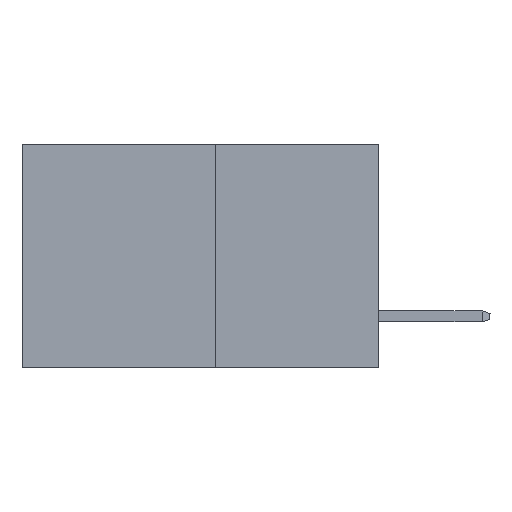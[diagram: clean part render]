
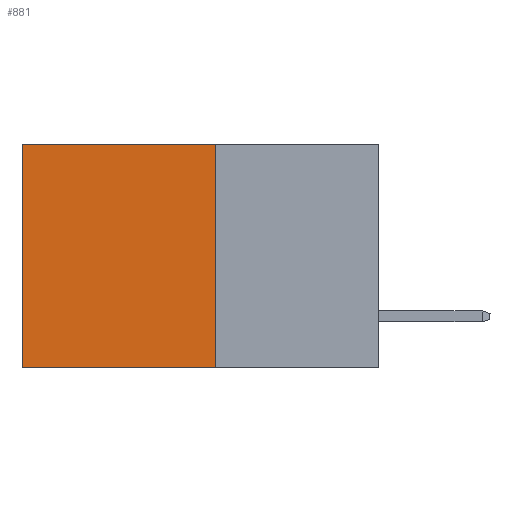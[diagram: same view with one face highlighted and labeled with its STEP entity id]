
A CAD part, left-side view. The second image highlights one B-rep face of the part: STEP entity #881.
In plain terms, the highlighted planar face has unit normal (-1, 0, 0).
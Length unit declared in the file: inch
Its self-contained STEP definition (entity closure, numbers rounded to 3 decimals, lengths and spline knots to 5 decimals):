
#537 = DIRECTION ( 'NONE',  ( 1., 0., 0. ) ) ;
#881 = ADVANCED_FACE ( 'NONE', ( #5533 ), #4506, .F. ) ;
#900 = VECTOR ( 'NONE', #11477, 39.37008 ) ;
#2496 = CARTESIAN_POINT ( 'NONE',  ( 0.277, 0.27, 0. ) ) ;
#2973 = DIRECTION ( 'NONE',  ( 0., 0., -1. ) ) ;
#3085 = DIRECTION ( 'NONE',  ( 0., 0., -1. ) ) ;
#3534 = CARTESIAN_POINT ( 'NONE',  ( 0.277, 0.27, -0.37 ) ) ;
#3695 = ORIENTED_EDGE ( 'NONE', *, *, #5024, .F. ) ;
#3900 = DIRECTION ( 'NONE',  ( 0., 1., 0. ) ) ;
#4506 = PLANE ( 'NONE',  #8404 ) ;
#4558 = CARTESIAN_POINT ( 'NONE',  ( 0.277, 0.27, -0.37 ) ) ;
#5024 = EDGE_CURVE ( 'NONE', #14234, #10140, #5389, .T. ) ;
#5389 = LINE ( 'NONE', #3534, #8649 ) ;
#5533 = FACE_OUTER_BOUND ( 'NONE', #7253, .T. ) ;
#6162 = CARTESIAN_POINT ( 'NONE',  ( 0.277, 0.59, 0. ) ) ;
#6541 = EDGE_CURVE ( 'NONE', #10140, #6581, #16179, .T. ) ;
#6581 = VERTEX_POINT ( 'NONE', #10130 ) ;
#7253 = EDGE_LOOP ( 'NONE', ( #15551, #8063, #3695, #11910 ) ) ;
#8063 = ORIENTED_EDGE ( 'NONE', *, *, #6541, .F. ) ;
#8404 = AXIS2_PLACEMENT_3D ( 'NONE', #4558, #537, #2973 ) ;
#8595 = CARTESIAN_POINT ( 'NONE',  ( 0.277, 0.59, -0.37 ) ) ;
#8649 = VECTOR ( 'NONE', #3085, 39.37008 ) ;
#9406 = EDGE_CURVE ( 'NONE', #14234, #10474, #9484, .T. ) ;
#9484 = LINE ( 'NONE', #2496, #16100 ) ;
#9980 = DIRECTION ( 'NONE',  ( 0., 0., -1. ) ) ;
#10130 = CARTESIAN_POINT ( 'NONE',  ( 0.277, 0.59, -0.37 ) ) ;
#10140 = VERTEX_POINT ( 'NONE', #13617 ) ;
#10474 = VERTEX_POINT ( 'NONE', #6162 ) ;
#11477 = DIRECTION ( 'NONE',  ( 0., 1., 0. ) ) ;
#11517 = EDGE_CURVE ( 'NONE', #10474, #6581, #13441, .T. ) ;
#11769 = CARTESIAN_POINT ( 'NONE',  ( 0.277, 0.27, -0.37 ) ) ;
#11910 = ORIENTED_EDGE ( 'NONE', *, *, #9406, .T. ) ;
#13042 = VECTOR ( 'NONE', #9980, 39.37008 ) ;
#13441 = LINE ( 'NONE', #8595, #13042 ) ;
#13617 = CARTESIAN_POINT ( 'NONE',  ( 0.277, 0.27, -0.37 ) ) ;
#14234 = VERTEX_POINT ( 'NONE', #15702 ) ;
#15551 = ORIENTED_EDGE ( 'NONE', *, *, #11517, .T. ) ;
#15702 = CARTESIAN_POINT ( 'NONE',  ( 0.277, 0.27, 0. ) ) ;
#16100 = VECTOR ( 'NONE', #3900, 39.37008 ) ;
#16179 = LINE ( 'NONE', #11769, #900 ) ;
